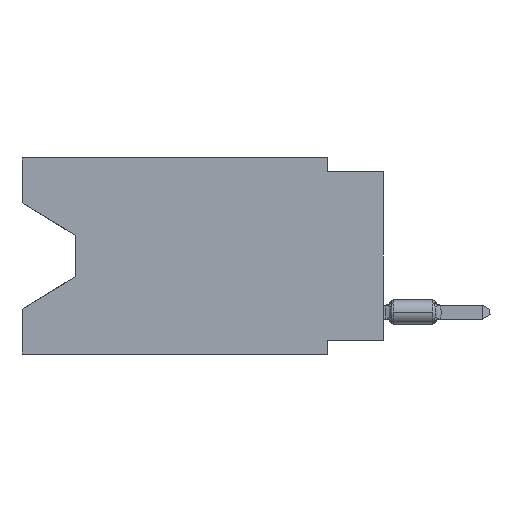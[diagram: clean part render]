
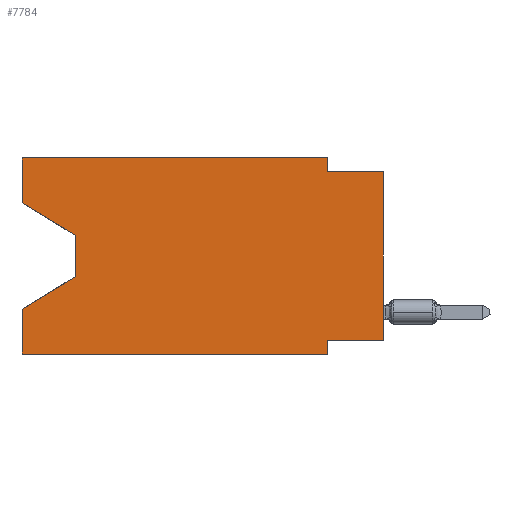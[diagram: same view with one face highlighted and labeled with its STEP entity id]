
A CAD part, left-side view. The second image highlights one B-rep face of the part: STEP entity #7784.
In plain terms, the highlighted planar face has unit normal (-1, 0, 0).
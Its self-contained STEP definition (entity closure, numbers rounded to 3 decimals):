
#1984 = DIRECTION ( 'NONE',  ( 0., -0.855, -0.519 ) ) ;
#2146 = EDGE_CURVE ( 'NONE', #89795, #40303, #48493, .T. ) ;
#3541 = EDGE_CURVE ( 'NONE', #87193, #62349, #47701, .T. ) ;
#6080 = ORIENTED_EDGE ( 'NONE', *, *, #11540, .F. ) ;
#6400 = CARTESIAN_POINT ( 'NONE',  ( 0., 16.383, 0. ) ) ;
#6567 = CARTESIAN_POINT ( 'NONE',  ( 0., 0., -0.635 ) ) ;
#7174 = DIRECTION ( 'NONE',  ( 0., 0., 1. ) ) ;
#7784 = ADVANCED_FACE ( 'NONE', ( #85970 ), #21118, .F. ) ;
#11540 = EDGE_CURVE ( 'NONE', #22977, #29097, #13870, .T. ) ;
#12463 = DIRECTION ( 'NONE',  ( 0., 0., -1. ) ) ;
#13870 = LINE ( 'NONE', #70239, #39790 ) ;
#14157 = VECTOR ( 'NONE', #7174, 1000. ) ;
#14960 = EDGE_CURVE ( 'NONE', #81810, #90086, #86453, .T. ) ;
#16907 = CARTESIAN_POINT ( 'NONE',  ( 0., 16.383, 0. ) ) ;
#16927 = DIRECTION ( 'NONE',  ( 0., 0., -1. ) ) ;
#16934 = DIRECTION ( 'NONE',  ( 0., 0.855, -0.519 ) ) ;
#18291 = CARTESIAN_POINT ( 'NONE',  ( 0., 0., -8.255 ) ) ;
#19609 = VECTOR ( 'NONE', #57245, 1000. ) ;
#19696 = EDGE_CURVE ( 'NONE', #40303, #29097, #24032, .T. ) ;
#20176 = CARTESIAN_POINT ( 'NONE',  ( 0., 16.383, 0. ) ) ;
#20256 = LINE ( 'NONE', #49181, #62950 ) ;
#20502 = DIRECTION ( 'NONE',  ( 0., 0., 1. ) ) ;
#21118 = PLANE ( 'NONE',  #45293 ) ;
#21599 = CARTESIAN_POINT ( 'NONE',  ( 0., 0., 0. ) ) ;
#21960 = VECTOR ( 'NONE', #69439, 1000. ) ;
#22977 = VERTEX_POINT ( 'NONE', #47723 ) ;
#23309 = VECTOR ( 'NONE', #85585, 1000. ) ;
#24032 = LINE ( 'NONE', #52958, #52883 ) ;
#27377 = CARTESIAN_POINT ( 'NONE',  ( 0., 16.383, -8.89 ) ) ;
#28646 = VECTOR ( 'NONE', #1984, 1000. ) ;
#28751 = ORIENTED_EDGE ( 'NONE', *, *, #59518, .F. ) ;
#29097 = VERTEX_POINT ( 'NONE', #30952 ) ;
#29321 = ORIENTED_EDGE ( 'NONE', *, *, #82744, .F. ) ;
#30675 = LINE ( 'NONE', #81795, #61691 ) ;
#30952 = CARTESIAN_POINT ( 'NONE',  ( 0., 16.383, -6.852 ) ) ;
#34430 = DIRECTION ( 'NONE',  ( 0., 0., 1. ) ) ;
#35316 = ORIENTED_EDGE ( 'NONE', *, *, #86239, .T. ) ;
#35555 = ORIENTED_EDGE ( 'NONE', *, *, #80895, .T. ) ;
#38590 = CARTESIAN_POINT ( 'NONE',  ( 0., 16.383, -2.038 ) ) ;
#39790 = VECTOR ( 'NONE', #20502, 1000. ) ;
#40303 = VERTEX_POINT ( 'NONE', #42039 ) ;
#41327 = EDGE_CURVE ( 'NONE', #57682, #87193, #44130, .T. ) ;
#41538 = DIRECTION ( 'NONE',  ( 1., 0., 0. ) ) ;
#42039 = CARTESIAN_POINT ( 'NONE',  ( 0., 13.97, -5.385 ) ) ;
#43169 = VECTOR ( 'NONE', #12463, 1000. ) ;
#43535 = VECTOR ( 'NONE', #86220, 1000. ) ;
#44130 = LINE ( 'NONE', #86708, #14157 ) ;
#44471 = ORIENTED_EDGE ( 'NONE', *, *, #19696, .T. ) ;
#45293 = AXIS2_PLACEMENT_3D ( 'NONE', #20176, #41538, #57594 ) ;
#45642 = ORIENTED_EDGE ( 'NONE', *, *, #3541, .F. ) ;
#46490 = LINE ( 'NONE', #89530, #28646 ) ;
#47701 = LINE ( 'NONE', #16907, #21960 ) ;
#47723 = CARTESIAN_POINT ( 'NONE',  ( 0., 16.383, -8.89 ) ) ;
#48493 = LINE ( 'NONE', #63137, #43169 ) ;
#49181 = CARTESIAN_POINT ( 'NONE',  ( 0., 2.54, -8.89 ) ) ;
#52883 = VECTOR ( 'NONE', #16934, 1000. ) ;
#52958 = CARTESIAN_POINT ( 'NONE',  ( 0., 13.97, -5.385 ) ) ;
#53940 = EDGE_LOOP ( 'NONE', ( #35316, #55012, #44471, #6080, #35555, #29321, #28751, #69138, #74575, #64669, #45642, #60212 ) ) ;
#55012 = ORIENTED_EDGE ( 'NONE', *, *, #2146, .T. ) ;
#57245 = DIRECTION ( 'NONE',  ( 0., -1., 0. ) ) ;
#57594 = DIRECTION ( 'NONE',  ( 0., 0., -1. ) ) ;
#57682 = VERTEX_POINT ( 'NONE', #38590 ) ;
#59518 = EDGE_CURVE ( 'NONE', #81810, #67459, #72471, .T. ) ;
#60212 = ORIENTED_EDGE ( 'NONE', *, *, #41327, .F. ) ;
#60303 = VERTEX_POINT ( 'NONE', #84133 ) ;
#61691 = VECTOR ( 'NONE', #16927, 1000. ) ;
#62349 = VERTEX_POINT ( 'NONE', #92240 ) ;
#62950 = VECTOR ( 'NONE', #86514, 1000. ) ;
#63022 = VECTOR ( 'NONE', #34430, 1000. ) ;
#63137 = CARTESIAN_POINT ( 'NONE',  ( 0., 13.97, -3.505 ) ) ;
#63535 = VERTEX_POINT ( 'NONE', #75246 ) ;
#64669 = ORIENTED_EDGE ( 'NONE', *, *, #65098, .F. ) ;
#65098 = EDGE_CURVE ( 'NONE', #62349, #63535, #30675, .T. ) ;
#67459 = VERTEX_POINT ( 'NONE', #74765 ) ;
#68960 = EDGE_CURVE ( 'NONE', #63535, #90086, #77239, .T. ) ;
#69138 = ORIENTED_EDGE ( 'NONE', *, *, #14960, .T. ) ;
#69439 = DIRECTION ( 'NONE',  ( 0., -1., 0. ) ) ;
#70239 = CARTESIAN_POINT ( 'NONE',  ( 0., 16.383, 0. ) ) ;
#72471 = LINE ( 'NONE', #86681, #43535 ) ;
#74575 = ORIENTED_EDGE ( 'NONE', *, *, #68960, .F. ) ;
#74765 = CARTESIAN_POINT ( 'NONE',  ( 0., 2.54, -8.255 ) ) ;
#75246 = CARTESIAN_POINT ( 'NONE',  ( 0., 2.54, -0.635 ) ) ;
#77239 = LINE ( 'NONE', #6567, #19609 ) ;
#80559 = CARTESIAN_POINT ( 'NONE',  ( 0., 0., -0.635 ) ) ;
#80895 = EDGE_CURVE ( 'NONE', #22977, #60303, #89893, .T. ) ;
#81795 = CARTESIAN_POINT ( 'NONE',  ( 0., 2.54, 0. ) ) ;
#81810 = VERTEX_POINT ( 'NONE', #18291 ) ;
#82744 = EDGE_CURVE ( 'NONE', #67459, #60303, #20256, .T. ) ;
#84133 = CARTESIAN_POINT ( 'NONE',  ( 0., 2.54, -8.89 ) ) ;
#85585 = DIRECTION ( 'NONE',  ( 0., -1., 0. ) ) ;
#85970 = FACE_OUTER_BOUND ( 'NONE', #53940, .T. ) ;
#86220 = DIRECTION ( 'NONE',  ( 0., 1., 0. ) ) ;
#86239 = EDGE_CURVE ( 'NONE', #57682, #89795, #46490, .T. ) ;
#86453 = LINE ( 'NONE', #21599, #63022 ) ;
#86514 = DIRECTION ( 'NONE',  ( 0., 0., -1. ) ) ;
#86681 = CARTESIAN_POINT ( 'NONE',  ( 0., 0., -8.255 ) ) ;
#86708 = CARTESIAN_POINT ( 'NONE',  ( 0., 16.383, 0. ) ) ;
#87193 = VERTEX_POINT ( 'NONE', #6400 ) ;
#89530 = CARTESIAN_POINT ( 'NONE',  ( 0., 16.383, -2.038 ) ) ;
#89647 = CARTESIAN_POINT ( 'NONE',  ( 0., 13.97, -3.505 ) ) ;
#89795 = VERTEX_POINT ( 'NONE', #89647 ) ;
#89893 = LINE ( 'NONE', #27377, #23309 ) ;
#90086 = VERTEX_POINT ( 'NONE', #80559 ) ;
#92240 = CARTESIAN_POINT ( 'NONE',  ( 0., 2.54, 0. ) ) ;
